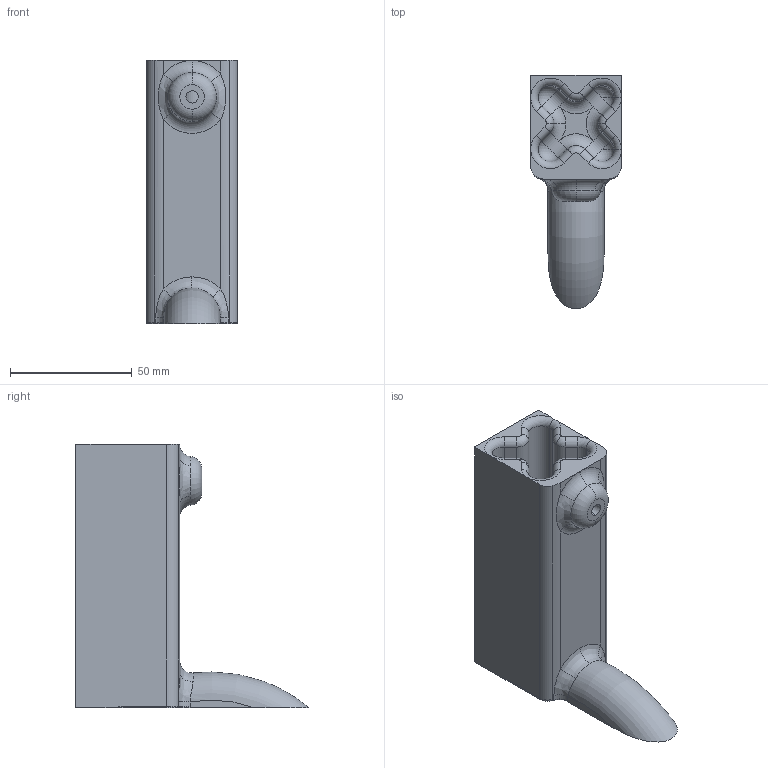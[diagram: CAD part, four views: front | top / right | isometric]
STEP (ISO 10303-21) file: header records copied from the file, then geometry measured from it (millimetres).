
FILE_DESCRIPTION (( 'STEP AP214' ), '1' );
FILE_NAME ('Charon_V3_Carbine_2.STEP', '2013-09-01T16:56:55', ( 'Asher' ), ( '' ), 'SwSTEP 2.0', 'SolidWorks 2013', '' );
FILE_SCHEMA (( 'AUTOMOTIVE_DESIGN' ));
Length unit declared in the file: millimetre
Products named in the file (1): Charon_V3_Carbine_2
Bounding box: 37.13 x 95.67 x 108 mm (x, y, z)
Volume: 113827 mm3; surface area: 36927.9 mm2
Topology: 1 solids, 1 shells, 166 faces, 507 edges, 299 vertices
Faces by surface type: sphere 72, cylinder 36, torus 23, plane 23, bspline 12
Entity records: 5702 total; most frequent: CARTESIAN_POINT 1819, DIRECTION 896, ORIENTED_EDGE 742, AXIS2_PLACEMENT_3D 407, EDGE_CURVE 371, CIRCLE 252, VERTEX_POINT 247, EDGE_LOOP 208
